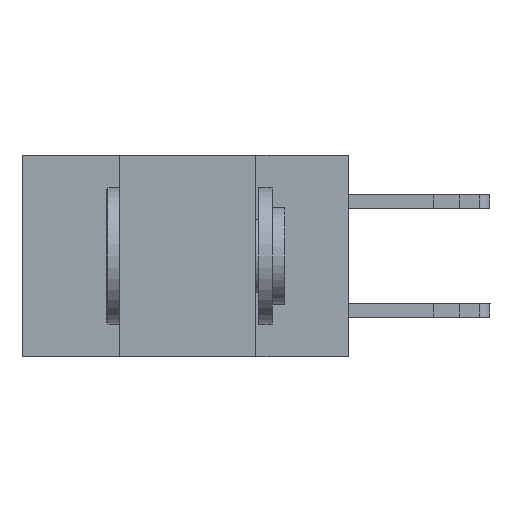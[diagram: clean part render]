
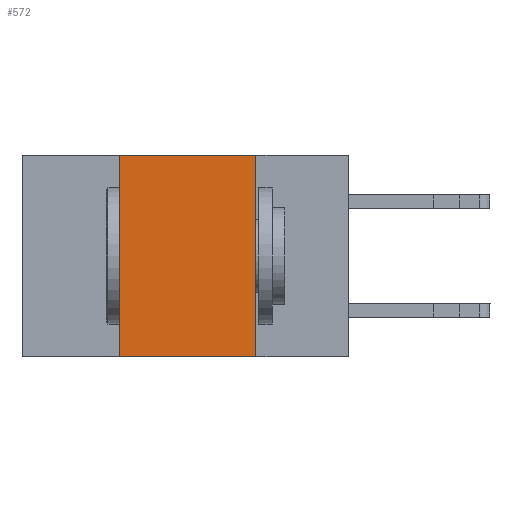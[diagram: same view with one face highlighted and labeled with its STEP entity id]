
A CAD part, left-side view. The second image highlights one B-rep face of the part: STEP entity #572.
In plain terms, the highlighted planar face has unit normal (-1, 0, 0).
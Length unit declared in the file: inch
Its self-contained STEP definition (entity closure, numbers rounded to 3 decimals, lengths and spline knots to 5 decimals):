
#272 = PLANE ( 'NONE',  #8464 ) ;
#336 = VECTOR ( 'NONE', #12170, 39.37008 ) ;
#525 = FACE_OUTER_BOUND ( 'NONE', #15570, .T. ) ;
#572 = ADVANCED_FACE ( 'NONE', ( #525 ), #272, .F. ) ;
#971 = CARTESIAN_POINT ( 'NONE',  ( 0., 0.17, -0.37 ) ) ;
#3472 = CARTESIAN_POINT ( 'NONE',  ( 0., 0.42, 0. ) ) ;
#4430 = EDGE_CURVE ( 'NONE', #11120, #10580, #17163, .T. ) ;
#4851 = EDGE_CURVE ( 'NONE', #11120, #15908, #6840, .T. ) ;
#6112 = DIRECTION ( 'NONE',  ( 0., -1., 0. ) ) ;
#6135 = CARTESIAN_POINT ( 'NONE',  ( 0., 0.6, -0.37 ) ) ;
#6476 = DIRECTION ( 'NONE',  ( 0., 0., -1. ) ) ;
#6569 = CARTESIAN_POINT ( 'NONE',  ( 0., 0.17, -0.37 ) ) ;
#6840 = LINE ( 'NONE', #6135, #18151 ) ;
#7319 = EDGE_CURVE ( 'NONE', #10580, #12477, #19803, .T. ) ;
#8464 = AXIS2_PLACEMENT_3D ( 'NONE', #12032, #17720, #6476 ) ;
#8681 = DIRECTION ( 'NONE',  ( 0., -1., 0. ) ) ;
#9084 = CARTESIAN_POINT ( 'NONE',  ( 0., 0.6, 0. ) ) ;
#9505 = CARTESIAN_POINT ( 'NONE',  ( 0., 0.17, 0. ) ) ;
#10580 = VERTEX_POINT ( 'NONE', #3472 ) ;
#11120 = VERTEX_POINT ( 'NONE', #11302 ) ;
#11298 = ORIENTED_EDGE ( 'NONE', *, *, #4430, .F. ) ;
#11302 = CARTESIAN_POINT ( 'NONE',  ( 0., 0.42, -0.37 ) ) ;
#11603 = EDGE_CURVE ( 'NONE', #12477, #15908, #16211, .T. ) ;
#11913 = VECTOR ( 'NONE', #15655, 39.37008 ) ;
#12032 = CARTESIAN_POINT ( 'NONE',  ( 0., 0.6, 0. ) ) ;
#12130 = CARTESIAN_POINT ( 'NONE',  ( 0., 0.42, -0.37 ) ) ;
#12170 = DIRECTION ( 'NONE',  ( 0., 0., 1. ) ) ;
#12477 = VERTEX_POINT ( 'NONE', #9505 ) ;
#13076 = ORIENTED_EDGE ( 'NONE', *, *, #7319, .F. ) ;
#13854 = ORIENTED_EDGE ( 'NONE', *, *, #4851, .T. ) ;
#15324 = ORIENTED_EDGE ( 'NONE', *, *, #11603, .F. ) ;
#15570 = EDGE_LOOP ( 'NONE', ( #15324, #13076, #11298, #13854 ) ) ;
#15655 = DIRECTION ( 'NONE',  ( 0., 0., -1. ) ) ;
#15908 = VERTEX_POINT ( 'NONE', #6569 ) ;
#16211 = LINE ( 'NONE', #971, #11913 ) ;
#17163 = LINE ( 'NONE', #12130, #336 ) ;
#17720 = DIRECTION ( 'NONE',  ( 1., 0., 0. ) ) ;
#18151 = VECTOR ( 'NONE', #6112, 39.37008 ) ;
#18300 = VECTOR ( 'NONE', #8681, 39.37008 ) ;
#19803 = LINE ( 'NONE', #9084, #18300 ) ;
